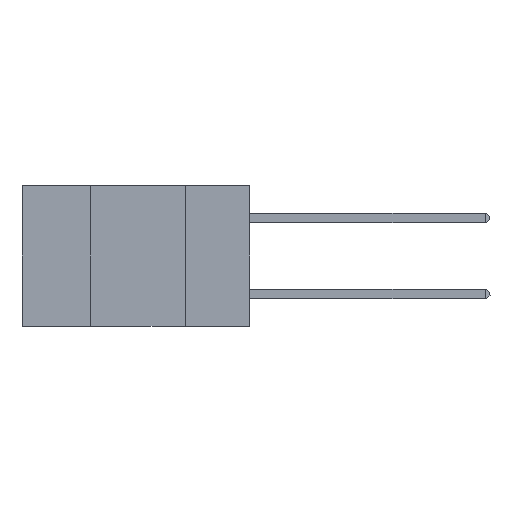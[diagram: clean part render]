
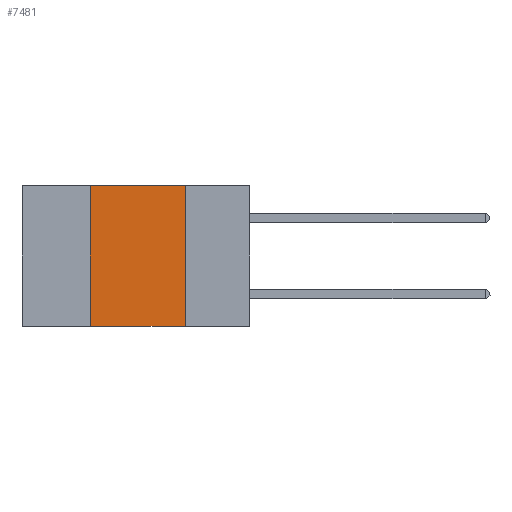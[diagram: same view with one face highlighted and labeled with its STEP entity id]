
A CAD part, left-side view. The second image highlights one B-rep face of the part: STEP entity #7481.
In plain terms, the highlighted planar face has unit normal (-1, 0, 0).
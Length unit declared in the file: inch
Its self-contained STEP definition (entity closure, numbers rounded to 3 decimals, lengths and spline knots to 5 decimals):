
#290 = AXIS2_PLACEMENT_3D ( 'NONE', #424, #9583, #8425 ) ;
#316 = FACE_OUTER_BOUND ( 'NONE', #2421, .T. ) ;
#424 = CARTESIAN_POINT ( 'NONE',  ( 0., 0.6, 0. ) ) ;
#588 = PLANE ( 'NONE',  #290 ) ;
#800 = VECTOR ( 'NONE', #7579, 39.37008 ) ;
#1313 = EDGE_CURVE ( 'NONE', #7988, #10923, #7444, .T. ) ;
#1363 = CARTESIAN_POINT ( 'NONE',  ( 0., 0.6, -0.37 ) ) ;
#1572 = VERTEX_POINT ( 'NONE', #5837 ) ;
#2001 = ORIENTED_EDGE ( 'NONE', *, *, #1313, .F. ) ;
#2050 = CARTESIAN_POINT ( 'NONE',  ( 0., 0.17, 0. ) ) ;
#2421 = EDGE_LOOP ( 'NONE', ( #6008, #2001, #12559, #3913 ) ) ;
#3464 = LINE ( 'NONE', #1363, #4245 ) ;
#3616 = LINE ( 'NONE', #12719, #800 ) ;
#3913 = ORIENTED_EDGE ( 'NONE', *, *, #6368, .T. ) ;
#4245 = VECTOR ( 'NONE', #4527, 39.37008 ) ;
#4527 = DIRECTION ( 'NONE',  ( 0., -1., 0. ) ) ;
#4840 = EDGE_CURVE ( 'NONE', #1572, #7988, #12292, .T. ) ;
#5426 = DIRECTION ( 'NONE',  ( 0., 0., 1. ) ) ;
#5780 = CARTESIAN_POINT ( 'NONE',  ( 0., 0.42, 0. ) ) ;
#5837 = CARTESIAN_POINT ( 'NONE',  ( 0., 0.42, -0.37 ) ) ;
#6008 = ORIENTED_EDGE ( 'NONE', *, *, #11871, .F. ) ;
#6368 = EDGE_CURVE ( 'NONE', #1572, #6739, #3464, .T. ) ;
#6612 = CARTESIAN_POINT ( 'NONE',  ( 0., 0.6, 0. ) ) ;
#6739 = VERTEX_POINT ( 'NONE', #8058 ) ;
#7444 = LINE ( 'NONE', #6612, #12621 ) ;
#7481 = ADVANCED_FACE ( 'NONE', ( #316 ), #588, .F. ) ;
#7579 = DIRECTION ( 'NONE',  ( 0., 0., -1. ) ) ;
#7988 = VERTEX_POINT ( 'NONE', #5780 ) ;
#8058 = CARTESIAN_POINT ( 'NONE',  ( 0., 0.17, -0.37 ) ) ;
#8425 = DIRECTION ( 'NONE',  ( 0., 0., -1. ) ) ;
#8526 = CARTESIAN_POINT ( 'NONE',  ( 0., 0.42, 0. ) ) ;
#9583 = DIRECTION ( 'NONE',  ( 1., 0., 0. ) ) ;
#9585 = DIRECTION ( 'NONE',  ( 0., -1., 0. ) ) ;
#10923 = VERTEX_POINT ( 'NONE', #2050 ) ;
#11871 = EDGE_CURVE ( 'NONE', #10923, #6739, #3616, .T. ) ;
#11966 = VECTOR ( 'NONE', #5426, 39.37008 ) ;
#12292 = LINE ( 'NONE', #8526, #11966 ) ;
#12559 = ORIENTED_EDGE ( 'NONE', *, *, #4840, .F. ) ;
#12621 = VECTOR ( 'NONE', #9585, 39.37008 ) ;
#12719 = CARTESIAN_POINT ( 'NONE',  ( 0., 0.17, 0. ) ) ;
